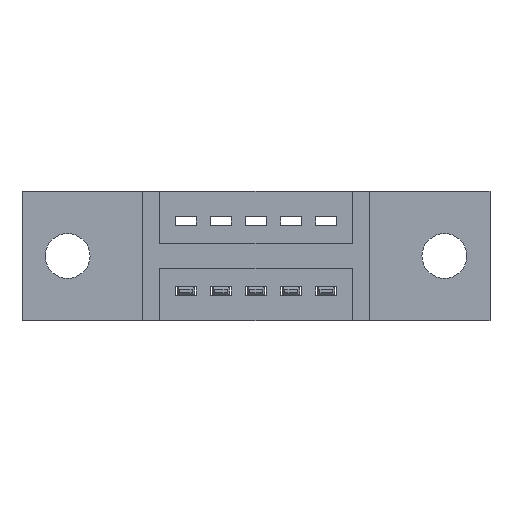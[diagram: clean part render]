
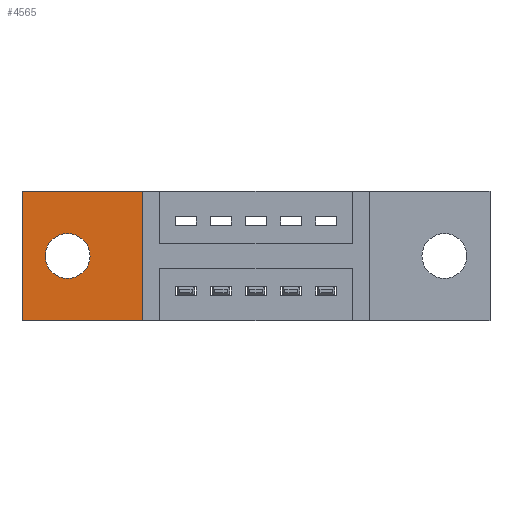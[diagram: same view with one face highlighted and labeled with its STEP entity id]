
A CAD part, front view. The second image highlights one B-rep face of the part: STEP entity #4565.
In plain terms, the highlighted planar face has unit normal (0, -1, 0).
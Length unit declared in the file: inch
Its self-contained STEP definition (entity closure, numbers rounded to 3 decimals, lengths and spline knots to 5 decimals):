
#265 = LINE ( 'NONE', #1226, #6936 ) ;
#440 = VERTEX_POINT ( 'NONE', #2130 ) ;
#550 = VERTEX_POINT ( 'NONE', #6377 ) ;
#578 = DIRECTION ( 'NONE',  ( 0., -1., 0. ) ) ;
#634 = AXIS2_PLACEMENT_3D ( 'NONE', #5705, #7731, #3973 ) ;
#1026 = EDGE_CURVE ( 'NONE', #3456, #440, #1437, .T. ) ;
#1226 = CARTESIAN_POINT ( 'NONE',  ( 0., 0.11, 0. ) ) ;
#1264 = ORIENTED_EDGE ( 'NONE', *, *, #5183, .T. ) ;
#1352 = VECTOR ( 'NONE', #5179, 39.37008 ) ;
#1437 = CIRCLE ( 'NONE', #2622, 0.064 ) ;
#1487 = ORIENTED_EDGE ( 'NONE', *, *, #4917, .T. ) ;
#1643 = ORIENTED_EDGE ( 'NONE', *, *, #1026, .F. ) ;
#1818 = CARTESIAN_POINT ( 'NONE',  ( 0.13, 0.11, -0.249 ) ) ;
#1840 = ORIENTED_EDGE ( 'NONE', *, *, #3061, .T. ) ;
#1855 = DIRECTION ( 'NONE',  ( 0., -1., 0. ) ) ;
#2130 = CARTESIAN_POINT ( 'NONE',  ( 0.13, 0.11, -0.121 ) ) ;
#2313 = DIRECTION ( 'NONE',  ( 0., 0., -1. ) ) ;
#2541 = CARTESIAN_POINT ( 'NONE',  ( 0., 0.11, -0.37 ) ) ;
#2622 = AXIS2_PLACEMENT_3D ( 'NONE', #8464, #1855, #5113 ) ;
#3061 = EDGE_CURVE ( 'NONE', #6072, #5270, #7349, .T. ) ;
#3225 = FACE_OUTER_BOUND ( 'NONE', #7892, .T. ) ;
#3350 = CARTESIAN_POINT ( 'NONE',  ( 0.3425, 0.11, -0.37 ) ) ;
#3363 = EDGE_CURVE ( 'NONE', #440, #3456, #3861, .T. ) ;
#3456 = VERTEX_POINT ( 'NONE', #1818 ) ;
#3513 = ORIENTED_EDGE ( 'NONE', *, *, #3363, .F. ) ;
#3674 = ORIENTED_EDGE ( 'NONE', *, *, #5564, .T. ) ;
#3719 = LINE ( 'NONE', #7762, #1352 ) ;
#3861 = CIRCLE ( 'NONE', #6390, 0.064 ) ;
#3973 = DIRECTION ( 'NONE',  ( 0., 0., -1. ) ) ;
#3976 = VECTOR ( 'NONE', #8007, 39.37008 ) ;
#4053 = VECTOR ( 'NONE', #5253, 39.37008 ) ;
#4335 = PLANE ( 'NONE',  #634 ) ;
#4565 = ADVANCED_FACE ( 'NONE', ( #5454, #3225 ), #4335, .T. ) ;
#4917 = EDGE_CURVE ( 'NONE', #4976, #6072, #5571, .T. ) ;
#4976 = VERTEX_POINT ( 'NONE', #6937 ) ;
#5113 = DIRECTION ( 'NONE',  ( 0., 0., -1. ) ) ;
#5179 = DIRECTION ( 'NONE',  ( -1., 0., 0. ) ) ;
#5183 = EDGE_CURVE ( 'NONE', #5270, #550, #3719, .T. ) ;
#5253 = DIRECTION ( 'NONE',  ( 1., 0., 0. ) ) ;
#5270 = VERTEX_POINT ( 'NONE', #7995 ) ;
#5454 = FACE_BOUND ( 'NONE', #6151, .T. ) ;
#5564 = EDGE_CURVE ( 'NONE', #550, #4976, #265, .T. ) ;
#5571 = LINE ( 'NONE', #2541, #4053 ) ;
#5705 = CARTESIAN_POINT ( 'NONE',  ( 0., 0.11, -0.37 ) ) ;
#6072 = VERTEX_POINT ( 'NONE', #3350 ) ;
#6151 = EDGE_LOOP ( 'NONE', ( #3513, #1643 ) ) ;
#6287 = DIRECTION ( 'NONE',  ( 0., 0., -1. ) ) ;
#6377 = CARTESIAN_POINT ( 'NONE',  ( 0., 0.11, 0. ) ) ;
#6390 = AXIS2_PLACEMENT_3D ( 'NONE', #8103, #578, #6287 ) ;
#6936 = VECTOR ( 'NONE', #2313, 39.37008 ) ;
#6937 = CARTESIAN_POINT ( 'NONE',  ( 0., 0.11, -0.37 ) ) ;
#7349 = LINE ( 'NONE', #7717, #3976 ) ;
#7717 = CARTESIAN_POINT ( 'NONE',  ( 0.3425, 0.11, 0. ) ) ;
#7731 = DIRECTION ( 'NONE',  ( 0., -1., 0. ) ) ;
#7762 = CARTESIAN_POINT ( 'NONE',  ( 0., 0.11, 0. ) ) ;
#7892 = EDGE_LOOP ( 'NONE', ( #3674, #1487, #1840, #1264 ) ) ;
#7995 = CARTESIAN_POINT ( 'NONE',  ( 0.3425, 0.11, 0. ) ) ;
#8007 = DIRECTION ( 'NONE',  ( 0., 0., 1. ) ) ;
#8103 = CARTESIAN_POINT ( 'NONE',  ( 0.13, 0.11, -0.185 ) ) ;
#8464 = CARTESIAN_POINT ( 'NONE',  ( 0.13, 0.11, -0.185 ) ) ;
